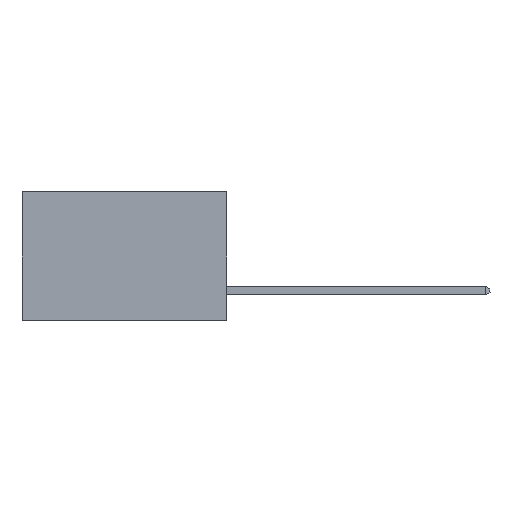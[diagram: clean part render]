
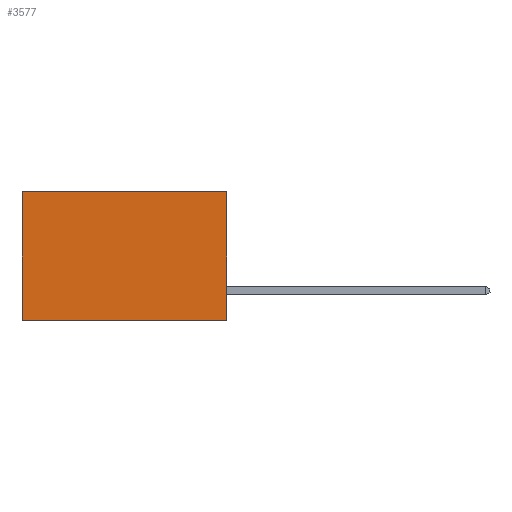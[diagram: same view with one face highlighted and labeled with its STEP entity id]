
A CAD part, left-side view. The second image highlights one B-rep face of the part: STEP entity #3577.
In plain terms, the highlighted planar face has unit normal (-1, 0, 0).
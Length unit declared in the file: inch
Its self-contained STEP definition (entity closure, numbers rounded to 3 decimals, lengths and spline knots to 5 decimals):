
#76 = LINE ( 'NONE', #471, #8323 ) ;
#85 = DIRECTION ( 'NONE',  ( 0., 0., -1. ) ) ;
#194 = DIRECTION ( 'NONE',  ( 0., 0., -1. ) ) ;
#305 = VERTEX_POINT ( 'NONE', #5436 ) ;
#471 = CARTESIAN_POINT ( 'NONE',  ( 0.277, 0., 0. ) ) ;
#734 = VERTEX_POINT ( 'NONE', #7291 ) ;
#748 = FACE_OUTER_BOUND ( 'NONE', #5399, .T. ) ;
#821 = CARTESIAN_POINT ( 'NONE',  ( 0.277, 0.59, -0.37 ) ) ;
#1201 = DIRECTION ( 'NONE',  ( 0., 1., 0. ) ) ;
#1409 = CARTESIAN_POINT ( 'NONE',  ( 0.277, 0., -0.37 ) ) ;
#1600 = ORIENTED_EDGE ( 'NONE', *, *, #5026, .F. ) ;
#1681 = VERTEX_POINT ( 'NONE', #7819 ) ;
#1826 = PLANE ( 'NONE',  #5933 ) ;
#2070 = EDGE_CURVE ( 'NONE', #734, #305, #3853, .T. ) ;
#2481 = ORIENTED_EDGE ( 'NONE', *, *, #7882, .T. ) ;
#3577 = ADVANCED_FACE ( 'NONE', ( #748 ), #1826, .F. ) ;
#3811 = VECTOR ( 'NONE', #5618, 39.37008 ) ;
#3853 = LINE ( 'NONE', #821, #4070 ) ;
#3990 = VECTOR ( 'NONE', #194, 39.37008 ) ;
#4070 = VECTOR ( 'NONE', #85, 39.37008 ) ;
#4112 = ORIENTED_EDGE ( 'NONE', *, *, #7629, .F. ) ;
#4808 = CARTESIAN_POINT ( 'NONE',  ( 0.277, 0., -0.37 ) ) ;
#4981 = DIRECTION ( 'NONE',  ( 0., 0., -1. ) ) ;
#5026 = EDGE_CURVE ( 'NONE', #5864, #305, #5550, .T. ) ;
#5092 = CARTESIAN_POINT ( 'NONE',  ( 0.277, 0., -0.37 ) ) ;
#5399 = EDGE_LOOP ( 'NONE', ( #6633, #1600, #4112, #2481 ) ) ;
#5436 = CARTESIAN_POINT ( 'NONE',  ( 0.277, 0.59, -0.37 ) ) ;
#5550 = LINE ( 'NONE', #5901, #3811 ) ;
#5618 = DIRECTION ( 'NONE',  ( 0., 1., 0. ) ) ;
#5674 = DIRECTION ( 'NONE',  ( 1., 0., 0. ) ) ;
#5864 = VERTEX_POINT ( 'NONE', #1409 ) ;
#5901 = CARTESIAN_POINT ( 'NONE',  ( 0.277, 0., -0.37 ) ) ;
#5933 = AXIS2_PLACEMENT_3D ( 'NONE', #4808, #5674, #4981 ) ;
#6633 = ORIENTED_EDGE ( 'NONE', *, *, #2070, .T. ) ;
#6884 = LINE ( 'NONE', #5092, #3990 ) ;
#7291 = CARTESIAN_POINT ( 'NONE',  ( 0.277, 0.59, 0. ) ) ;
#7629 = EDGE_CURVE ( 'NONE', #1681, #5864, #6884, .T. ) ;
#7819 = CARTESIAN_POINT ( 'NONE',  ( 0.277, 0., 0. ) ) ;
#7882 = EDGE_CURVE ( 'NONE', #1681, #734, #76, .T. ) ;
#8323 = VECTOR ( 'NONE', #1201, 39.37008 ) ;
